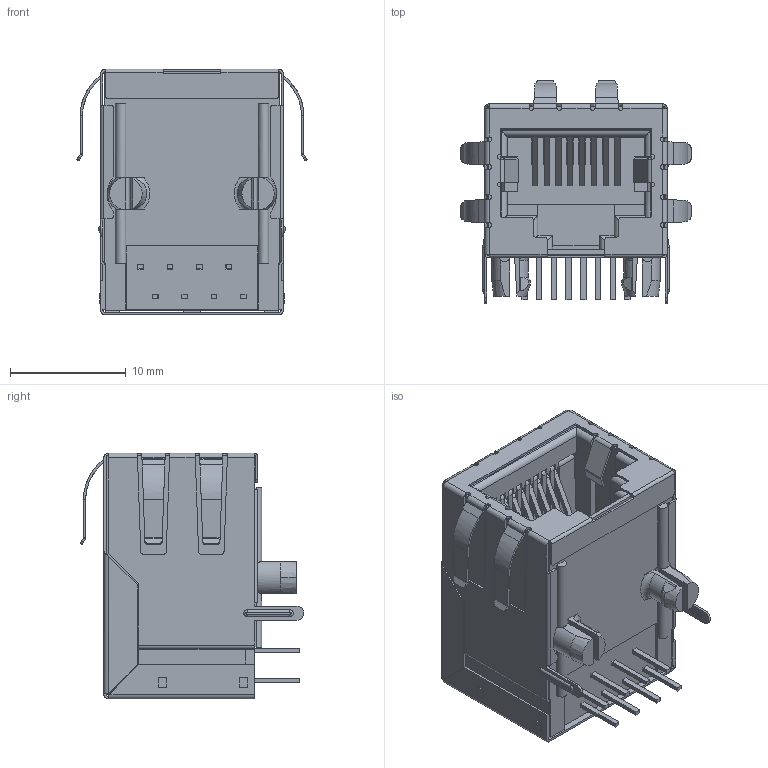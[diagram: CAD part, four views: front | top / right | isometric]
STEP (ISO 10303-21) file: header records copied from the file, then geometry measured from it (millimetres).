
FILE_DESCRIPTION (( 'STEP AP203' ), '1' );
FILE_NAME ('J9P018892N00201.STEP', '2020-03-20T01:17:42', ( '' ), ( '' ), 'SwSTEP 2.0', 'SolidWorks 2016', '' );
FILE_SCHEMA (( 'CONFIG_CONTROL_DESIGN' ));
Length unit declared in the file: millimetre
Products named in the file (6): 9P-NOLED Contacts; 9P-NOLED Shield; 9P-NOLED Assembly; 9P-NOLED Insulator; J9P018892N00201; 9P-NOLED Contact Lock
Assembly tree (5 placements, depth 3):
  J9P018892N00201
    9P-NOLED Assembly
      9P-NOLED Insulator
      9P-NOLED Contacts
      9P-NOLED Contact Lock
      9P-NOLED Shield
Bounding box: 19.9 x 19.36 x 21.25 mm (x, y, z)
Volume: 2583.4 mm3; surface area: 7121.4 mm2
Topology: 11 solids, 11 shells, 1313 faces, 3375 edges, 2057 vertices
Faces by surface type: plane 892, cylinder 319, bspline 61, cone 39, torus 2
Entity records: 42700 total; most frequent: CARTESIAN_POINT 11632, ORIENTED_EDGE 6750, DIRECTION 5599, EDGE_CURVE 3375, VECTOR 2437, LINE 2437, VERTEX_POINT 2057, AXIS2_PLACEMENT_3D 1581
